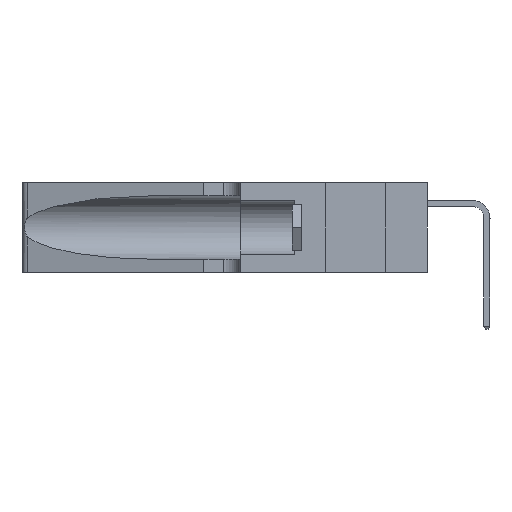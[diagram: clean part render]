
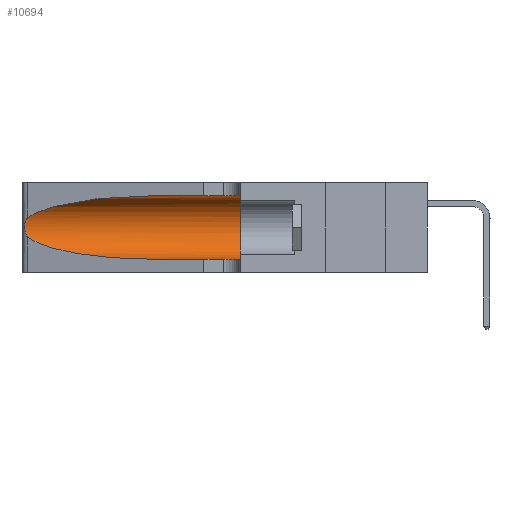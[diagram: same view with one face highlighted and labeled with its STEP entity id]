
A CAD part, left-side view. The second image highlights one B-rep face of the part: STEP entity #10694.
In plain terms, the highlighted cylindrical face has radius 3.308 mm (diameter 6.617 mm), a partial arc.
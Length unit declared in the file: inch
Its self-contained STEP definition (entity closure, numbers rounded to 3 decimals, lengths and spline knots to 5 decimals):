
#1177 = CARTESIAN_POINT ( 'NONE',  ( 0.25487, 1.22718, 0.14631 ) ) ;
#2649 = CARTESIAN_POINT ( 'NONE',  ( 0.1305, 0.72297, 0.31525 ) ) ;
#3508 = EDGE_CURVE ( 'NONE', #18851, #17157, #37253, .T. ) ;
#4174 = CARTESIAN_POINT ( 'NONE',  ( 0.25639, 1.23184, 0.21858 ) ) ;
#4740 = ORIENTED_EDGE ( 'NONE', *, *, #22821, .T. ) ;
#5147 = CARTESIAN_POINT ( 'NONE',  ( 0.1305, 0.72297, 0.05475 ) ) ;
#6030 = DIRECTION ( 'NONE',  ( 0., -1., 0. ) ) ;
#6102 = DIRECTION ( 'NONE',  ( 0., -1., 0. ) ) ;
#6674 = VERTEX_POINT ( 'NONE', #22547 ) ;
#7030 = ORIENTED_EDGE ( 'NONE', *, *, #18439, .F. ) ;
#7209 =( BOUNDED_CURVE ( )  B_SPLINE_CURVE ( 3, ( #2649, #14974, #32321, #35238 ),
 .UNSPECIFIED., .F., .F. ) 
 B_SPLINE_CURVE_WITH_KNOTS ( ( 4, 4 ),
 ( 1.5708, 2.84003 ),
 .UNSPECIFIED. ) 
 CURVE ( )  GEOMETRIC_REPRESENTATION_ITEM ( )  RATIONAL_B_SPLINE_CURVE ( ( 1., 0.87, 0.87, 1. ) ) 
 REPRESENTATION_ITEM ( '' )  );
#7264 = CARTESIAN_POINT ( 'NONE',  ( 0.25854, 1.2359, 0.20912 ) ) ;
#7602 = CARTESIAN_POINT ( 'NONE',  ( 0.25487, 1.22718, 0.22369 ) ) ;
#7724 = CYLINDRICAL_SURFACE ( 'NONE', #9564, 0.13025 ) ;
#9249 = VECTOR ( 'NONE', #6102, 39.37008 ) ;
#9564 = AXIS2_PLACEMENT_3D ( 'NONE', #30224, #33079, #18697 ) ;
#10369 = CARTESIAN_POINT ( 'NONE',  ( 0.26075, 1.23896, 0.19203 ) ) ;
#10694 = ADVANCED_FACE ( 'NONE', ( #23635 ), #7724, .F. ) ;
#12427 = CARTESIAN_POINT ( 'NONE',  ( 0.1305, 0.35, 0.185 ) ) ;
#13253 = AXIS2_PLACEMENT_3D ( 'NONE', #12427, #32799, #15471 ) ;
#13396 = CARTESIAN_POINT ( 'NONE',  ( 0.26017, 1.23833, 0.17102 ) ) ;
#13595 = ORIENTED_EDGE ( 'NONE', *, *, #17662, .T. ) ;
#13811 = VERTEX_POINT ( 'NONE', #18008 ) ;
#14689 = B_SPLINE_CURVE_WITH_KNOTS ( 'NONE', 3,
 ( #33600, #22294, #4174, #25146, #7264, #28006, #10369, #30862, #13396, #33732, #16482, #36663, #19495, #1177 ),
 .UNSPECIFIED., .F., .F.,
 ( 4, 2, 2, 2, 2, 2, 4 ),
 ( 0., 0.00027, 0.00053, 0.00107, 0.0016, 0.00187, 0.00214 ),
 .UNSPECIFIED. ) ;
#14974 = CARTESIAN_POINT ( 'NONE',  ( 0.18966, 0.96281, 0.31525 ) ) ;
#15000 = ORIENTED_EDGE ( 'NONE', *, *, #19683, .T. ) ;
#15193 = CARTESIAN_POINT ( 'NONE',  ( 0.1305, 1.61858, 0.31525 ) ) ;
#15471 = DIRECTION ( 'NONE',  ( 0., 0., 1. ) ) ;
#16482 = CARTESIAN_POINT ( 'NONE',  ( 0.25789, 1.23486, 0.15765 ) ) ;
#17157 = VERTEX_POINT ( 'NONE', #27420 ) ;
#17662 = EDGE_CURVE ( 'NONE', #35594, #26900, #7209, .T. ) ;
#18008 = CARTESIAN_POINT ( 'NONE',  ( 0.1305, 0.35, 0.05475 ) ) ;
#18439 = EDGE_CURVE ( 'NONE', #35594, #6674, #25047, .T. ) ;
#18697 = DIRECTION ( 'NONE',  ( 0., 0., -1. ) ) ;
#18851 = VERTEX_POINT ( 'NONE', #28423 ) ;
#19495 = CARTESIAN_POINT ( 'NONE',  ( 0.25555, 1.22993, 0.14849 ) ) ;
#19683 = EDGE_CURVE ( 'NONE', #17157, #13811, #31200, .T. ) ;
#20294 = CARTESIAN_POINT ( 'NONE',  ( 0.2373, 1.15595, 0.08982 ) ) ;
#22294 = CARTESIAN_POINT ( 'NONE',  ( 0.25555, 1.22994, 0.2215 ) ) ;
#22547 = CARTESIAN_POINT ( 'NONE',  ( 0.1305, 0.35, 0.31525 ) ) ;
#22821 = EDGE_CURVE ( 'NONE', #26900, #18851, #14689, .T. ) ;
#23174 = CARTESIAN_POINT ( 'NONE',  ( 0.25487, 1.22718, 0.14631 ) ) ;
#23635 = FACE_OUTER_BOUND ( 'NONE', #29643, .T. ) ;
#25047 = LINE ( 'NONE', #15193, #9249 ) ;
#25146 = CARTESIAN_POINT ( 'NONE',  ( 0.25787, 1.23484, 0.2124 ) ) ;
#25220 = CARTESIAN_POINT ( 'NONE',  ( 0.1305, 0.72297, 0.31525 ) ) ;
#26900 = VERTEX_POINT ( 'NONE', #7602 ) ;
#27420 = CARTESIAN_POINT ( 'NONE',  ( 0.1305, 0.72297, 0.05475 ) ) ;
#28006 = CARTESIAN_POINT ( 'NONE',  ( 0.26018, 1.23835, 0.19895 ) ) ;
#28423 = CARTESIAN_POINT ( 'NONE',  ( 0.25487, 1.22718, 0.14631 ) ) ;
#28800 = CARTESIAN_POINT ( 'NONE',  ( 0.18966, 0.96281, 0.05475 ) ) ;
#29261 = ORIENTED_EDGE ( 'NONE', *, *, #29802, .F. ) ;
#29643 = EDGE_LOOP ( 'NONE', ( #13595, #4740, #30621, #15000, #29261, #7030 ) ) ;
#29802 = EDGE_CURVE ( 'NONE', #6674, #13811, #33161, .T. ) ;
#30224 = CARTESIAN_POINT ( 'NONE',  ( 0.1305, 1.61858, 0.185 ) ) ;
#30621 = ORIENTED_EDGE ( 'NONE', *, *, #3508, .T. ) ;
#30862 = CARTESIAN_POINT ( 'NONE',  ( 0.26075, 1.23896, 0.178 ) ) ;
#31200 = LINE ( 'NONE', #32445, #37079 ) ;
#32321 = CARTESIAN_POINT ( 'NONE',  ( 0.2373, 1.15595, 0.28018 ) ) ;
#32445 = CARTESIAN_POINT ( 'NONE',  ( 0.1305, 1.61858, 0.05475 ) ) ;
#32799 = DIRECTION ( 'NONE',  ( 0., 1., 0. ) ) ;
#33079 = DIRECTION ( 'NONE',  ( 0., -1., 0. ) ) ;
#33161 = CIRCLE ( 'NONE', #13253, 0.13025 ) ;
#33600 = CARTESIAN_POINT ( 'NONE',  ( 0.25487, 1.22718, 0.22369 ) ) ;
#33732 = CARTESIAN_POINT ( 'NONE',  ( 0.25856, 1.23593, 0.16098 ) ) ;
#35238 = CARTESIAN_POINT ( 'NONE',  ( 0.25487, 1.22718, 0.22369 ) ) ;
#35594 = VERTEX_POINT ( 'NONE', #25220 ) ;
#36663 = CARTESIAN_POINT ( 'NONE',  ( 0.25639, 1.23186, 0.15144 ) ) ;
#37079 = VECTOR ( 'NONE', #6030, 39.37008 ) ;
#37253 =( BOUNDED_CURVE ( )  B_SPLINE_CURVE ( 3, ( #23174, #20294, #28800, #5147 ),
 .UNSPECIFIED., .F., .F. ) 
 B_SPLINE_CURVE_WITH_KNOTS ( ( 4, 4 ),
 ( 3.44316, 4.71239 ),
 .UNSPECIFIED. ) 
 CURVE ( )  GEOMETRIC_REPRESENTATION_ITEM ( )  RATIONAL_B_SPLINE_CURVE ( ( 1., 0.87, 0.87, 1. ) ) 
 REPRESENTATION_ITEM ( '' )  );
